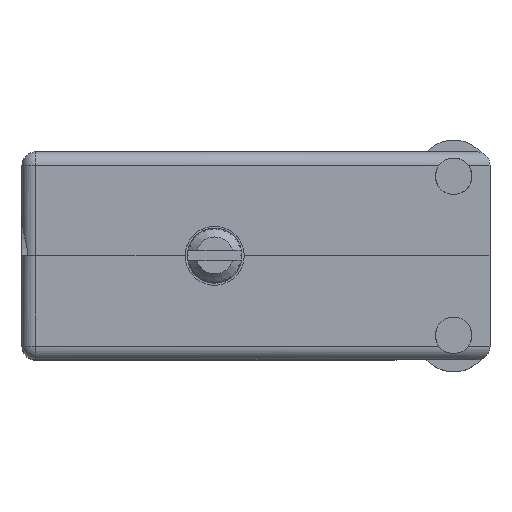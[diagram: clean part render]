
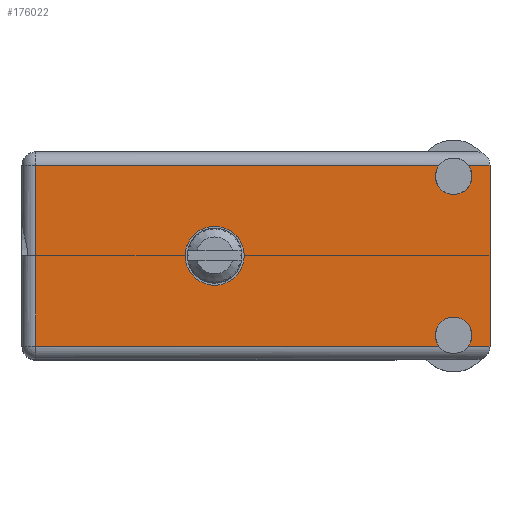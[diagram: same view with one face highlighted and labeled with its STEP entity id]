
A CAD part, top view. The second image highlights one B-rep face of the part: STEP entity #176022.
In plain terms, the highlighted face is planar.
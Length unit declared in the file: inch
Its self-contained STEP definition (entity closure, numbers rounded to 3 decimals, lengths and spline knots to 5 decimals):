
#6438 = CARTESIAN_POINT ( 'NONE',  ( 0.87187, 0.806, 0.3105 ) ) ;
#9616 = CARTESIAN_POINT ( 'NONE',  ( 0.8215, 0.806, -0.2735 ) ) ;
#18864 = VERTEX_POINT ( 'NONE', #53490 ) ;
#20803 = ORIENTED_EDGE ( 'NONE', *, *, #168505, .T. ) ;
#26684 = ORIENTED_EDGE ( 'NONE', *, *, #98710, .F. ) ;
#27293 = VECTOR ( 'NONE', #113756, 39.37008 ) ;
#27828 = CARTESIAN_POINT ( 'NONE',  ( 0.8215, 0.806, -0.2735 ) ) ;
#28798 = DIRECTION ( 'NONE',  ( 0., 1., 0. ) ) ;
#31198 = ORIENTED_EDGE ( 'NONE', *, *, #107615, .F. ) ;
#32859 = AXIS2_PLACEMENT_3D ( 'NONE', #121741, #78384, #107287 ) ;
#33356 = VERTEX_POINT ( 'NONE', #95898 ) ;
#33487 = ORIENTED_EDGE ( 'NONE', *, *, #122743, .F. ) ;
#34587 = CARTESIAN_POINT ( 'NONE',  ( 0.9465, 0.806, 0.3575 ) ) ;
#38436 = CARTESIAN_POINT ( 'NONE',  ( 0.8215, 0.806, -0.211 ) ) ;
#38481 = CARTESIAN_POINT ( 'NONE',  ( -0.6155, 0.806, 0.3105 ) ) ;
#39443 = DIRECTION ( 'NONE',  ( 0., 1., 0. ) ) ;
#42255 = CARTESIAN_POINT ( 'NONE',  ( 0.9465, 0.806, 0.3105 ) ) ;
#45482 = CARTESIAN_POINT ( 'NONE',  ( -0.6625, 0.806, -0.3575 ) ) ;
#48530 = EDGE_CURVE ( 'NONE', #171744, #161875, #107137, .T. ) ;
#49256 = EDGE_CURVE ( 'NONE', #161875, #54079, #164947, .T. ) ;
#50904 = DIRECTION ( 'NONE',  ( 0., 0., 1. ) ) ;
#52389 = EDGE_CURVE ( 'NONE', #84187, #54079, #85828, .T. ) ;
#53490 = CARTESIAN_POINT ( 'NONE',  ( 0., 0.806, 0.1015 ) ) ;
#54079 = VERTEX_POINT ( 'NONE', #143668 ) ;
#55497 = CARTESIAN_POINT ( 'NONE',  ( 0.8215, 0.806, 0.211 ) ) ;
#55557 = VECTOR ( 'NONE', #115727, 39.37008 ) ;
#55791 = DIRECTION ( 'NONE',  ( 0., 0., 1. ) ) ;
#57087 = PLANE ( 'NONE',  #156928 ) ;
#58107 = DIRECTION ( 'NONE',  ( 0., 0., 1. ) ) ;
#58193 = ORIENTED_EDGE ( 'NONE', *, *, #111558, .T. ) ;
#59355 = ORIENTED_EDGE ( 'NONE', *, *, #140270, .F. ) ;
#62503 = CARTESIAN_POINT ( 'NONE',  ( 0.8215, 0.806, 0.2735 ) ) ;
#63799 = ORIENTED_EDGE ( 'NONE', *, *, #141227, .T. ) ;
#64067 = DIRECTION ( 'NONE',  ( -1., 0., 0. ) ) ;
#64391 = DIRECTION ( 'NONE',  ( 0., 1., 0. ) ) ;
#65293 = ORIENTED_EDGE ( 'NONE', *, *, #52389, .T. ) ;
#65321 = DIRECTION ( 'NONE',  ( 0., 1., 0. ) ) ;
#71463 = LINE ( 'NONE', #130180, #27293 ) ;
#71508 = DIRECTION ( 'NONE',  ( 0., 1., 0. ) ) ;
#71816 = CARTESIAN_POINT ( 'NONE',  ( 0.77113, 0.806, -0.3105 ) ) ;
#75384 = CARTESIAN_POINT ( 'NONE',  ( -0.6155, 0.806, -0.3105 ) ) ;
#76165 = ORIENTED_EDGE ( 'NONE', *, *, #48530, .F. ) ;
#78384 = DIRECTION ( 'NONE',  ( 0., 1., 0. ) ) ;
#80086 = ORIENTED_EDGE ( 'NONE', *, *, #112451, .T. ) ;
#84187 = VERTEX_POINT ( 'NONE', #38481 ) ;
#85388 = EDGE_LOOP ( 'NONE', ( #33487, #26684 ) ) ;
#85828 = LINE ( 'NONE', #188846, #55557 ) ;
#86048 = CARTESIAN_POINT ( 'NONE',  ( 0.9465, 0.806, -0.3105 ) ) ;
#86667 = CARTESIAN_POINT ( 'NONE',  ( -0.6155, 0.806, -0.3575 ) ) ;
#88560 = LINE ( 'NONE', #86667, #116614 ) ;
#88793 = FACE_BOUND ( 'NONE', #85388, .T. ) ;
#94634 = DIRECTION ( 'NONE',  ( -1., 0., 0. ) ) ;
#95898 = CARTESIAN_POINT ( 'NONE',  ( 0., 0.806, -0.1015 ) ) ;
#96291 = AXIS2_PLACEMENT_3D ( 'NONE', #27828, #28798, #142390 ) ;
#98710 = EDGE_CURVE ( 'NONE', #33356, #18864, #112679, .T. ) ;
#102631 = VECTOR ( 'NONE', #64067, 39.37008 ) ;
#106577 = VERTEX_POINT ( 'NONE', #86048 ) ;
#107137 = CIRCLE ( 'NONE', #113056, 0.0625 ) ;
#107287 = DIRECTION ( 'NONE',  ( 0., 0., 1. ) ) ;
#107615 = EDGE_CURVE ( 'NONE', #188069, #159290, #188515, .T. ) ;
#111558 = EDGE_CURVE ( 'NONE', #106577, #159290, #113396, .T. ) ;
#112451 = EDGE_CURVE ( 'NONE', #170541, #130837, #155220, .T. ) ;
#112679 = CIRCLE ( 'NONE', #32859, 0.1015 ) ;
#113056 = AXIS2_PLACEMENT_3D ( 'NONE', #189950, #144720, #58107 ) ;
#113396 = LINE ( 'NONE', #139093, #102631 ) ;
#113756 = DIRECTION ( 'NONE',  ( 1., 0., 0. ) ) ;
#115005 = ORIENTED_EDGE ( 'NONE', *, *, #49256, .F. ) ;
#115727 = DIRECTION ( 'NONE',  ( 1., 0., 0. ) ) ;
#116614 = VECTOR ( 'NONE', #145381, 39.37008 ) ;
#116774 = DIRECTION ( 'NONE',  ( -1., 0., 0. ) ) ;
#121339 = CIRCLE ( 'NONE', #182690, 0.1015 ) ;
#121741 = CARTESIAN_POINT ( 'NONE',  ( 0., 0.806, 0. ) ) ;
#122743 = EDGE_CURVE ( 'NONE', #18864, #33356, #121339, .T. ) ;
#125651 = AXIS2_PLACEMENT_3D ( 'NONE', #9616, #39443, #55791 ) ;
#127517 = CARTESIAN_POINT ( 'NONE',  ( 0.87187, 0.806, -0.3105 ) ) ;
#130180 = CARTESIAN_POINT ( 'NONE',  ( 0.9465, 0.806, 0.3105 ) ) ;
#130376 = VECTOR ( 'NONE', #94634, 39.37008 ) ;
#130837 = VERTEX_POINT ( 'NONE', #75384 ) ;
#136611 = DIRECTION ( 'NONE',  ( 0., 0., 1. ) ) ;
#137549 = CARTESIAN_POINT ( 'NONE',  ( 0., 0.806, 0. ) ) ;
#139093 = CARTESIAN_POINT ( 'NONE',  ( -0.6625, 0.806, -0.3105 ) ) ;
#140270 = EDGE_CURVE ( 'NONE', #170541, #188069, #174825, .T. ) ;
#141227 = EDGE_CURVE ( 'NONE', #171744, #141523, #71463, .T. ) ;
#141523 = VERTEX_POINT ( 'NONE', #42255 ) ;
#142390 = DIRECTION ( 'NONE',  ( 0., 0., 1. ) ) ;
#143668 = CARTESIAN_POINT ( 'NONE',  ( 0.77113, 0.806, 0.3105 ) ) ;
#144720 = DIRECTION ( 'NONE',  ( 0., 1., 0. ) ) ;
#145381 = DIRECTION ( 'NONE',  ( 0., 0., 1. ) ) ;
#145610 = FACE_OUTER_BOUND ( 'NONE', #172037, .T. ) ;
#155220 = LINE ( 'NONE', #183169, #130376 ) ;
#156928 = AXIS2_PLACEMENT_3D ( 'NONE', #45482, #71508, #116774 ) ;
#157885 = ORIENTED_EDGE ( 'NONE', *, *, #184982, .F. ) ;
#159290 = VERTEX_POINT ( 'NONE', #127517 ) ;
#160625 = VECTOR ( 'NONE', #50904, 39.37008 ) ;
#161875 = VERTEX_POINT ( 'NONE', #55497 ) ;
#164947 = CIRCLE ( 'NONE', #189523, 0.0625 ) ;
#167349 = DIRECTION ( 'NONE',  ( 0., 0., 1. ) ) ;
#168505 = EDGE_CURVE ( 'NONE', #130837, #84187, #88560, .T. ) ;
#170541 = VERTEX_POINT ( 'NONE', #71816 ) ;
#171744 = VERTEX_POINT ( 'NONE', #6438 ) ;
#172037 = EDGE_LOOP ( 'NONE', ( #65293, #115005, #76165, #63799, #157885, #58193, #31198, #59355, #80086, #20803 ) ) ;
#174825 = CIRCLE ( 'NONE', #125651, 0.0625 ) ;
#176022 = ADVANCED_FACE ( 'NONE', ( #88793, #145610 ), #57087, .T. ) ;
#182690 = AXIS2_PLACEMENT_3D ( 'NONE', #137549, #64391, #136611 ) ;
#182753 = LINE ( 'NONE', #34587, #160625 ) ;
#183169 = CARTESIAN_POINT ( 'NONE',  ( -0.6625, 0.806, -0.3105 ) ) ;
#184982 = EDGE_CURVE ( 'NONE', #106577, #141523, #182753, .T. ) ;
#188069 = VERTEX_POINT ( 'NONE', #38436 ) ;
#188515 = CIRCLE ( 'NONE', #96291, 0.0625 ) ;
#188846 = CARTESIAN_POINT ( 'NONE',  ( 0.9465, 0.806, 0.3105 ) ) ;
#189523 = AXIS2_PLACEMENT_3D ( 'NONE', #62503, #65321, #167349 ) ;
#189950 = CARTESIAN_POINT ( 'NONE',  ( 0.8215, 0.806, 0.2735 ) ) ;
